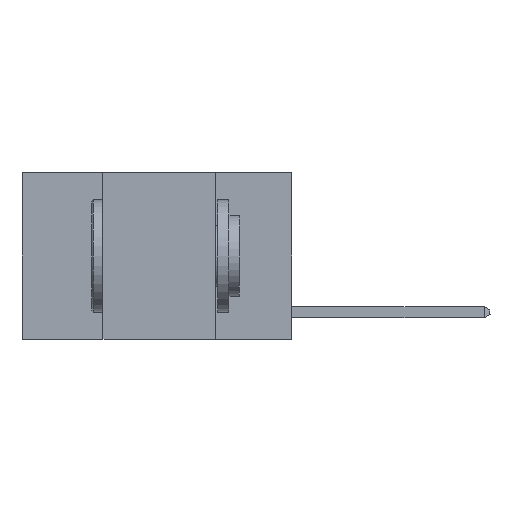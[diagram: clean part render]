
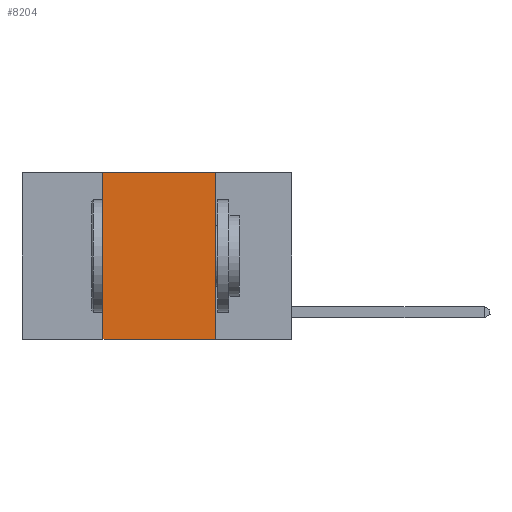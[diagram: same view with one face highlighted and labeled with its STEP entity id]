
A CAD part, left-side view. The second image highlights one B-rep face of the part: STEP entity #8204.
In plain terms, the highlighted planar face has unit normal (-1, 0, 0).
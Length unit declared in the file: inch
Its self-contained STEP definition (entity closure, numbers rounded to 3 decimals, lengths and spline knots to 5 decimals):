
#420 = EDGE_CURVE ( 'NONE', #20938, #14049, #2511, .T. ) ;
#490 = DIRECTION ( 'NONE',  ( 0., 0., 1. ) ) ;
#727 = CARTESIAN_POINT ( 'NONE',  ( 0., 0.6, 0. ) ) ;
#955 = PLANE ( 'NONE',  #16096 ) ;
#1626 = VECTOR ( 'NONE', #16972, 39.37008 ) ;
#2315 = LINE ( 'NONE', #15220, #18532 ) ;
#2511 = LINE ( 'NONE', #9782, #1626 ) ;
#3173 = DIRECTION ( 'NONE',  ( 0., -1., 0. ) ) ;
#3790 = VERTEX_POINT ( 'NONE', #19840 ) ;
#4099 = VECTOR ( 'NONE', #490, 39.37008 ) ;
#4341 = DIRECTION ( 'NONE',  ( 0., 0., -1. ) ) ;
#6385 = EDGE_CURVE ( 'NONE', #3790, #6509, #23039, .T. ) ;
#6509 = VERTEX_POINT ( 'NONE', #20774 ) ;
#8172 = CARTESIAN_POINT ( 'NONE',  ( 0., 0.17, 0. ) ) ;
#8204 = ADVANCED_FACE ( 'NONE', ( #18976 ), #955, .F. ) ;
#8585 = EDGE_LOOP ( 'NONE', ( #23162, #22271, #15965, #16259 ) ) ;
#9782 = CARTESIAN_POINT ( 'NONE',  ( 0., 0.6, 0. ) ) ;
#11307 = CARTESIAN_POINT ( 'NONE',  ( 0., 0.42, 0. ) ) ;
#13090 = LINE ( 'NONE', #11307, #4099 ) ;
#13371 = CARTESIAN_POINT ( 'NONE',  ( 0., 0.42, 0. ) ) ;
#14049 = VERTEX_POINT ( 'NONE', #8172 ) ;
#14068 = CARTESIAN_POINT ( 'NONE',  ( 0., 0.6, -0.37 ) ) ;
#15220 = CARTESIAN_POINT ( 'NONE',  ( 0., 0.17, 0. ) ) ;
#15965 = ORIENTED_EDGE ( 'NONE', *, *, #19865, .F. ) ;
#16096 = AXIS2_PLACEMENT_3D ( 'NONE', #727, #17095, #4341 ) ;
#16259 = ORIENTED_EDGE ( 'NONE', *, *, #6385, .T. ) ;
#16972 = DIRECTION ( 'NONE',  ( 0., -1., 0. ) ) ;
#17095 = DIRECTION ( 'NONE',  ( 1., 0., 0. ) ) ;
#18532 = VECTOR ( 'NONE', #18777, 39.37008 ) ;
#18777 = DIRECTION ( 'NONE',  ( 0., 0., -1. ) ) ;
#18976 = FACE_OUTER_BOUND ( 'NONE', #8585, .T. ) ;
#19409 = VECTOR ( 'NONE', #3173, 39.37008 ) ;
#19840 = CARTESIAN_POINT ( 'NONE',  ( 0., 0.42, -0.37 ) ) ;
#19865 = EDGE_CURVE ( 'NONE', #3790, #20938, #13090, .T. ) ;
#20774 = CARTESIAN_POINT ( 'NONE',  ( 0., 0.17, -0.37 ) ) ;
#20938 = VERTEX_POINT ( 'NONE', #13371 ) ;
#22271 = ORIENTED_EDGE ( 'NONE', *, *, #420, .F. ) ;
#22700 = EDGE_CURVE ( 'NONE', #14049, #6509, #2315, .T. ) ;
#23039 = LINE ( 'NONE', #14068, #19409 ) ;
#23162 = ORIENTED_EDGE ( 'NONE', *, *, #22700, .F. ) ;
